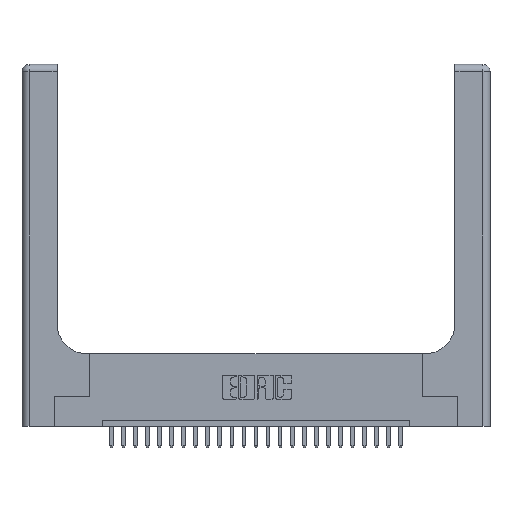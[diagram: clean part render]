
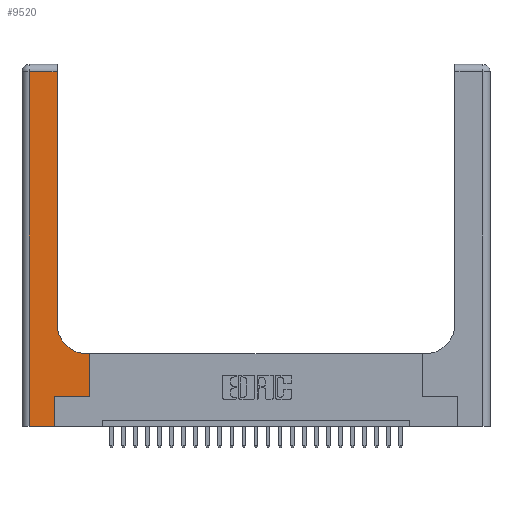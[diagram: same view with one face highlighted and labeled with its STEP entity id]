
A CAD part, top view. The second image highlights one B-rep face of the part: STEP entity #9520.
In plain terms, the highlighted planar face has unit normal (0, 0, 1).
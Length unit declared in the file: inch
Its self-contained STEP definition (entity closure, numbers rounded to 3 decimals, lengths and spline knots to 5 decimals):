
#25 = EDGE_LOOP ( 'NONE', ( #21856, #5586, #16573, #18462, #14980, #15132, #20048, #8247, #3932 ) ) ;
#1357 = DIRECTION ( 'NONE',  ( 0., 1., 0. ) ) ;
#2026 = FACE_OUTER_BOUND ( 'NONE', #25, .T. ) ;
#2272 = VERTEX_POINT ( 'NONE', #22791 ) ;
#2583 = DIRECTION ( 'NONE',  ( 0., 1., 0. ) ) ;
#3616 = CARTESIAN_POINT ( 'NONE',  ( 0., 2.94, 0.37 ) ) ;
#3623 = EDGE_CURVE ( 'NONE', #13027, #9163, #8634, .T. ) ;
#3674 = CARTESIAN_POINT ( 'NONE',  ( 0.06, 0., 0.37 ) ) ;
#3932 = ORIENTED_EDGE ( 'NONE', *, *, #18600, .T. ) ;
#5165 = LINE ( 'NONE', #21256, #15405 ) ;
#5337 = EDGE_CURVE ( 'NONE', #6136, #2272, #24211, .T. ) ;
#5586 = ORIENTED_EDGE ( 'NONE', *, *, #9079, .T. ) ;
#5736 = LINE ( 'NONE', #24779, #24227 ) ;
#5986 = CARTESIAN_POINT ( 'NONE',  ( 0.2915, 3., 0.37 ) ) ;
#6136 = VERTEX_POINT ( 'NONE', #23995 ) ;
#6144 = LINE ( 'NONE', #3616, #21776 ) ;
#6340 = CARTESIAN_POINT ( 'NONE',  ( 0.5585, 0.25, 0.37 ) ) ;
#6498 = LINE ( 'NONE', #5986, #20240 ) ;
#6513 = DIRECTION ( 'NONE',  ( 0., 0., -1. ) ) ;
#7066 = AXIS2_PLACEMENT_3D ( 'NONE', #18784, #6513, #12243 ) ;
#7524 = DIRECTION ( 'NONE',  ( 1., 0., 0. ) ) ;
#8247 = ORIENTED_EDGE ( 'NONE', *, *, #13567, .T. ) ;
#8267 = AXIS2_PLACEMENT_3D ( 'NONE', #12241, #26304, #14103 ) ;
#8377 = CARTESIAN_POINT ( 'NONE',  ( 0.06, 2.94, 0.37 ) ) ;
#8576 = CIRCLE ( 'NONE', #8267, 0.25 ) ;
#8634 = LINE ( 'NONE', #6340, #24224 ) ;
#8895 = CARTESIAN_POINT ( 'NONE',  ( 0.06, 3., 0.37 ) ) ;
#9050 = CARTESIAN_POINT ( 'NONE',  ( 0.2915, 2.94, 0.37 ) ) ;
#9079 = EDGE_CURVE ( 'NONE', #25345, #15794, #6144, .T. ) ;
#9163 = VERTEX_POINT ( 'NONE', #23830 ) ;
#9520 = ADVANCED_FACE ( 'NONE', ( #2026 ), #10749, .F. ) ;
#9648 = CARTESIAN_POINT ( 'NONE',  ( 0., 0., 0.37 ) ) ;
#9732 = VERTEX_POINT ( 'NONE', #18213 ) ;
#10749 = PLANE ( 'NONE',  #7066 ) ;
#12241 = CARTESIAN_POINT ( 'NONE',  ( 0.5415, 0.85, 0.37 ) ) ;
#12243 = DIRECTION ( 'NONE',  ( -1., 0., 0. ) ) ;
#12461 = EDGE_CURVE ( 'NONE', #24319, #25345, #6498, .T. ) ;
#13027 = VERTEX_POINT ( 'NONE', #20042 ) ;
#13032 = EDGE_CURVE ( 'NONE', #15794, #17555, #21490, .T. ) ;
#13397 = VECTOR ( 'NONE', #1357, 39.37008 ) ;
#13567 = EDGE_CURVE ( 'NONE', #9163, #9732, #5165, .T. ) ;
#14103 = DIRECTION ( 'NONE',  ( 1., 0., 0. ) ) ;
#14878 = LINE ( 'NONE', #9648, #25049 ) ;
#14980 = ORIENTED_EDGE ( 'NONE', *, *, #5337, .T. ) ;
#15132 = ORIENTED_EDGE ( 'NONE', *, *, #15390, .T. ) ;
#15142 = VECTOR ( 'NONE', #19223, 39.37008 ) ;
#15390 = EDGE_CURVE ( 'NONE', #2272, #13027, #5736, .T. ) ;
#15405 = VECTOR ( 'NONE', #17434, 39.37008 ) ;
#15794 = VERTEX_POINT ( 'NONE', #8377 ) ;
#16573 = ORIENTED_EDGE ( 'NONE', *, *, #13032, .T. ) ;
#17434 = DIRECTION ( 'NONE',  ( -1., 0., 0. ) ) ;
#17555 = VERTEX_POINT ( 'NONE', #3674 ) ;
#17694 = CARTESIAN_POINT ( 'NONE',  ( 0.269, 0., 0.37 ) ) ;
#17983 = DIRECTION ( 'NONE',  ( -1., 0., 0. ) ) ;
#18213 = CARTESIAN_POINT ( 'NONE',  ( 0.5415, 0.6, 0.37 ) ) ;
#18462 = ORIENTED_EDGE ( 'NONE', *, *, #20063, .T. ) ;
#18600 = EDGE_CURVE ( 'NONE', #9732, #24319, #8576, .T. ) ;
#18784 = CARTESIAN_POINT ( 'NONE',  ( 0., 3., 0.37 ) ) ;
#19223 = DIRECTION ( 'NONE',  ( 0., -1., 0. ) ) ;
#20042 = CARTESIAN_POINT ( 'NONE',  ( 0.5585, 0.25, 0.37 ) ) ;
#20048 = ORIENTED_EDGE ( 'NONE', *, *, #3623, .T. ) ;
#20063 = EDGE_CURVE ( 'NONE', #17555, #6136, #14878, .T. ) ;
#20240 = VECTOR ( 'NONE', #2583, 39.37008 ) ;
#20794 = DIRECTION ( 'NONE',  ( 1., 0., 0. ) ) ;
#21256 = CARTESIAN_POINT ( 'NONE',  ( 0.2915, 0.6, 0.37 ) ) ;
#21490 = LINE ( 'NONE', #8895, #15142 ) ;
#21530 = CARTESIAN_POINT ( 'NONE',  ( 0.2915, 0.85, 0.37 ) ) ;
#21776 = VECTOR ( 'NONE', #17983, 39.37008 ) ;
#21856 = ORIENTED_EDGE ( 'NONE', *, *, #12461, .T. ) ;
#22791 = CARTESIAN_POINT ( 'NONE',  ( 0.269, 0.25, 0.37 ) ) ;
#23830 = CARTESIAN_POINT ( 'NONE',  ( 0.5585, 0.6, 0.37 ) ) ;
#23995 = CARTESIAN_POINT ( 'NONE',  ( 0.269, 0., 0.37 ) ) ;
#24211 = LINE ( 'NONE', #17694, #13397 ) ;
#24224 = VECTOR ( 'NONE', #24316, 39.37008 ) ;
#24227 = VECTOR ( 'NONE', #20794, 39.37008 ) ;
#24316 = DIRECTION ( 'NONE',  ( 0., 1., 0. ) ) ;
#24319 = VERTEX_POINT ( 'NONE', #21530 ) ;
#24779 = CARTESIAN_POINT ( 'NONE',  ( 0.269, 0.25, 0.37 ) ) ;
#25049 = VECTOR ( 'NONE', #7524, 39.37008 ) ;
#25345 = VERTEX_POINT ( 'NONE', #9050 ) ;
#26304 = DIRECTION ( 'NONE',  ( 0., 0., -1. ) ) ;
